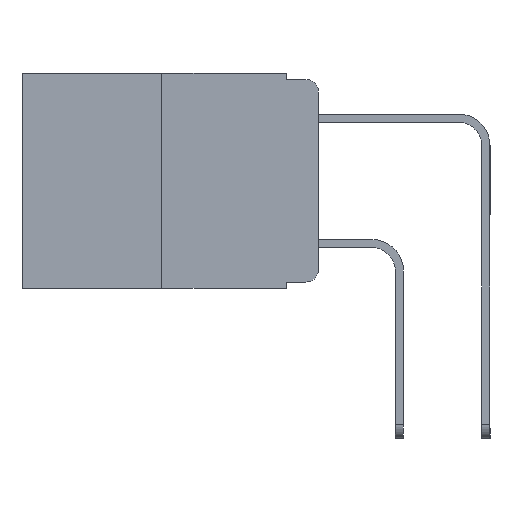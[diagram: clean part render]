
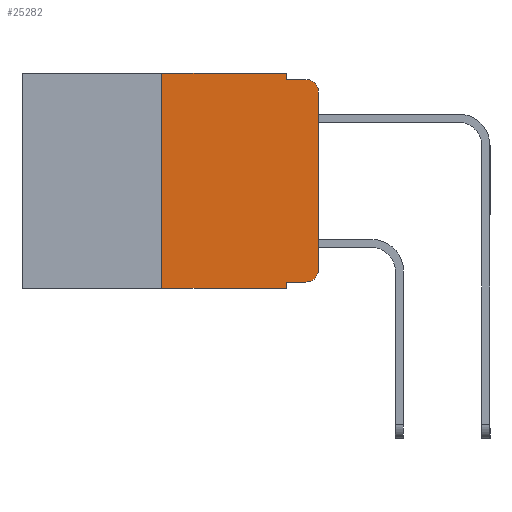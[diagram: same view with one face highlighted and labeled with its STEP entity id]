
A CAD part, left-side view. The second image highlights one B-rep face of the part: STEP entity #25282.
In plain terms, the highlighted planar face has unit normal (-1, 0, 0).
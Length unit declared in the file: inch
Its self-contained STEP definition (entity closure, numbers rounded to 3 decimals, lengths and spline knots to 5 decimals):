
#45 = EDGE_CURVE ( 'NONE', #5126, #22808, #3951, .T. ) ;
#55 = DIRECTION ( 'NONE',  ( 0., -1., 0. ) ) ;
#199 = DIRECTION ( 'NONE',  ( 0., 0., -1. ) ) ;
#453 = VERTEX_POINT ( 'NONE', #19174 ) ;
#653 = DIRECTION ( 'NONE',  ( -1., 0., 0. ) ) ;
#937 = CARTESIAN_POINT ( 'NONE',  ( 0., 0.051, -0.333 ) ) ;
#2051 = EDGE_CURVE ( 'NONE', #22808, #7962, #15628, .T. ) ;
#2358 = ORIENTED_EDGE ( 'NONE', *, *, #22282, .F. ) ;
#3003 = VECTOR ( 'NONE', #18550, 39.37008 ) ;
#3208 = ORIENTED_EDGE ( 'NONE', *, *, #3411, .F. ) ;
#3321 = DIRECTION ( 'NONE',  ( 0., 0., -1. ) ) ;
#3411 = EDGE_CURVE ( 'NONE', #7962, #22818, #16158, .T. ) ;
#3451 = PLANE ( 'NONE',  #19311 ) ;
#3646 = ORIENTED_EDGE ( 'NONE', *, *, #4712, .T. ) ;
#3803 = VERTEX_POINT ( 'NONE', #19280 ) ;
#3951 = LINE ( 'NONE', #5198, #24102 ) ;
#3977 = CARTESIAN_POINT ( 'NONE',  ( 0., 0.051, -0.01 ) ) ;
#4551 = ORIENTED_EDGE ( 'NONE', *, *, #21004, .T. ) ;
#4712 = EDGE_CURVE ( 'NONE', #9987, #22818, #4954, .T. ) ;
#4849 = CARTESIAN_POINT ( 'NONE',  ( 0., 0.25, 0. ) ) ;
#4910 = DIRECTION ( 'NONE',  ( 0., -1., 0. ) ) ;
#4954 = CIRCLE ( 'NONE', #11934, 0.02 ) ;
#5055 = CARTESIAN_POINT ( 'NONE',  ( 0., 0.051, -0.01 ) ) ;
#5126 = VERTEX_POINT ( 'NONE', #14522 ) ;
#5198 = CARTESIAN_POINT ( 'NONE',  ( 0., 0.473, 0. ) ) ;
#5589 = CARTESIAN_POINT ( 'NONE',  ( 0., 0.02, -0.333 ) ) ;
#5696 = FACE_OUTER_BOUND ( 'NONE', #17076, .T. ) ;
#5814 = VERTEX_POINT ( 'NONE', #24198 ) ;
#7104 = VECTOR ( 'NONE', #4910, 39.37008 ) ;
#7332 = EDGE_CURVE ( 'NONE', #453, #9987, #19880, .T. ) ;
#7520 = AXIS2_PLACEMENT_3D ( 'NONE', #12494, #653, #14476 ) ;
#7546 = VERTEX_POINT ( 'NONE', #5589 ) ;
#7650 = VECTOR ( 'NONE', #3321, 39.37008 ) ;
#7962 = VERTEX_POINT ( 'NONE', #5055 ) ;
#8516 = DIRECTION ( 'NONE',  ( 0., -1., 0. ) ) ;
#9132 = LINE ( 'NONE', #14815, #23520 ) ;
#9354 = CARTESIAN_POINT ( 'NONE',  ( 0., 0.473, 0. ) ) ;
#9435 = LINE ( 'NONE', #4849, #3003 ) ;
#9987 = VERTEX_POINT ( 'NONE', #14131 ) ;
#10154 = CARTESIAN_POINT ( 'NONE',  ( 0., 0.051, 0. ) ) ;
#10203 = CARTESIAN_POINT ( 'NONE',  ( 0., 0.02, -0.01 ) ) ;
#10699 = ORIENTED_EDGE ( 'NONE', *, *, #17438, .T. ) ;
#10826 = DIRECTION ( 'NONE',  ( 0., -1., 0. ) ) ;
#11265 = CARTESIAN_POINT ( 'NONE',  ( 0., 0.02, -0.03 ) ) ;
#11385 = DIRECTION ( 'NONE',  ( 0., 0., -1. ) ) ;
#11934 = AXIS2_PLACEMENT_3D ( 'NONE', #11265, #24833, #13255 ) ;
#12379 = LINE ( 'NONE', #937, #7104 ) ;
#12494 = CARTESIAN_POINT ( 'NONE',  ( 0., 0.02, -0.313 ) ) ;
#12898 = ORIENTED_EDGE ( 'NONE', *, *, #7332, .T. ) ;
#12943 = LINE ( 'NONE', #17123, #7650 ) ;
#13255 = DIRECTION ( 'NONE',  ( 0., 0., -1. ) ) ;
#13493 = ORIENTED_EDGE ( 'NONE', *, *, #19695, .T. ) ;
#14131 = CARTESIAN_POINT ( 'NONE',  ( 0., 0., -0.03 ) ) ;
#14199 = CARTESIAN_POINT ( 'NONE',  ( 0., 0.051, 0. ) ) ;
#14399 = ORIENTED_EDGE ( 'NONE', *, *, #45, .F. ) ;
#14476 = DIRECTION ( 'NONE',  ( 0., 0., -1. ) ) ;
#14522 = CARTESIAN_POINT ( 'NONE',  ( 0., 0.25, 0. ) ) ;
#14715 = VECTOR ( 'NONE', #20821, 39.37008 ) ;
#14815 = CARTESIAN_POINT ( 'NONE',  ( 0., 0.473, -0.343 ) ) ;
#15628 = LINE ( 'NONE', #10154, #20168 ) ;
#16158 = LINE ( 'NONE', #3977, #20716 ) ;
#16588 = ORIENTED_EDGE ( 'NONE', *, *, #23547, .F. ) ;
#16939 = CARTESIAN_POINT ( 'NONE',  ( 0., 0., 0. ) ) ;
#17076 = EDGE_LOOP ( 'NONE', ( #12898, #3646, #3208, #20241, #14399, #16588, #10699, #2358, #4551, #13493 ) ) ;
#17103 = CIRCLE ( 'NONE', #7520, 0.02 ) ;
#17123 = CARTESIAN_POINT ( 'NONE',  ( 0., 0.051, 0. ) ) ;
#17438 = EDGE_CURVE ( 'NONE', #24736, #3803, #9132, .T. ) ;
#18550 = DIRECTION ( 'NONE',  ( 0., 0., 1. ) ) ;
#19174 = CARTESIAN_POINT ( 'NONE',  ( 0., 0., -0.313 ) ) ;
#19280 = CARTESIAN_POINT ( 'NONE',  ( 0., 0.051, -0.343 ) ) ;
#19311 = AXIS2_PLACEMENT_3D ( 'NONE', #9354, #23059, #11385 ) ;
#19695 = EDGE_CURVE ( 'NONE', #7546, #453, #17103, .T. ) ;
#19880 = LINE ( 'NONE', #16939, #14715 ) ;
#20168 = VECTOR ( 'NONE', #199, 39.37008 ) ;
#20241 = ORIENTED_EDGE ( 'NONE', *, *, #2051, .F. ) ;
#20716 = VECTOR ( 'NONE', #55, 39.37008 ) ;
#20821 = DIRECTION ( 'NONE',  ( 0., 0., 1. ) ) ;
#21004 = EDGE_CURVE ( 'NONE', #5814, #7546, #12379, .T. ) ;
#22282 = EDGE_CURVE ( 'NONE', #5814, #3803, #12943, .T. ) ;
#22808 = VERTEX_POINT ( 'NONE', #14199 ) ;
#22818 = VERTEX_POINT ( 'NONE', #10203 ) ;
#23059 = DIRECTION ( 'NONE',  ( 1., 0., 0. ) ) ;
#23520 = VECTOR ( 'NONE', #10826, 39.37008 ) ;
#23547 = EDGE_CURVE ( 'NONE', #24736, #5126, #9435, .T. ) ;
#24102 = VECTOR ( 'NONE', #8516, 39.37008 ) ;
#24198 = CARTESIAN_POINT ( 'NONE',  ( 0., 0.051, -0.333 ) ) ;
#24736 = VERTEX_POINT ( 'NONE', #25214 ) ;
#24833 = DIRECTION ( 'NONE',  ( -1., 0., 0. ) ) ;
#25214 = CARTESIAN_POINT ( 'NONE',  ( 0., 0.25, -0.343 ) ) ;
#25282 = ADVANCED_FACE ( 'NONE', ( #5696 ), #3451, .F. ) ;
